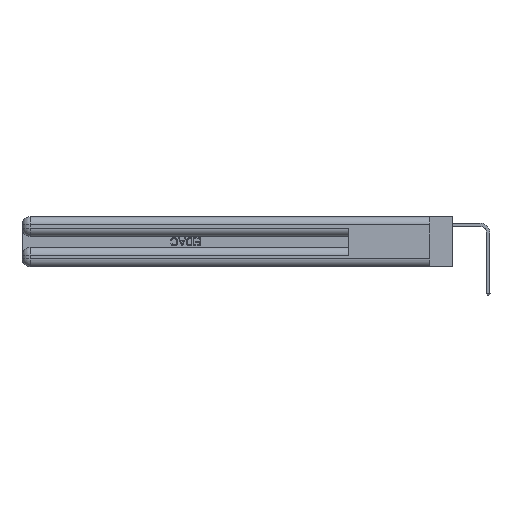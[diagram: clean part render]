
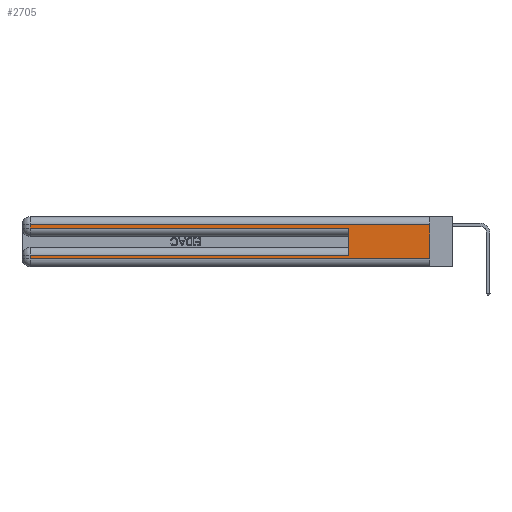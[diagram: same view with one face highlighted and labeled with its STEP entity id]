
A CAD part, left-side view. The second image highlights one B-rep face of the part: STEP entity #2705.
In plain terms, the highlighted planar face has unit normal (-1, 0, 0).
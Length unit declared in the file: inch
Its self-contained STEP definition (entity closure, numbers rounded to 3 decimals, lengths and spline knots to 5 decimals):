
#549 = LINE ( 'NONE', #13289, #26780 ) ;
#654 = CARTESIAN_POINT ( 'NONE',  ( 0., 0., 0.31 ) ) ;
#1462 = EDGE_CURVE ( 'NONE', #16318, #24122, #12923, .T. ) ;
#1870 = EDGE_LOOP ( 'NONE', ( #3384, #30017, #4647, #6444, #7582, #5738, #4512, #25020 ) ) ;
#2015 = EDGE_CURVE ( 'NONE', #24122, #26317, #24005, .T. ) ;
#2305 = VERTEX_POINT ( 'NONE', #14566 ) ;
#2485 = EDGE_CURVE ( 'NONE', #26317, #19376, #29432, .T. ) ;
#2705 = ADVANCED_FACE ( 'NONE', ( #11775 ), #16457, .F. ) ;
#2742 = VECTOR ( 'NONE', #7947, 39.37008 ) ;
#2922 = DIRECTION ( 'NONE',  ( 0., -1., 0. ) ) ;
#3250 = CARTESIAN_POINT ( 'NONE',  ( 0., 2.94, 0.37 ) ) ;
#3368 = CARTESIAN_POINT ( 'NONE',  ( 0., 0.6, 0.285 ) ) ;
#3384 = ORIENTED_EDGE ( 'NONE', *, *, #27199, .F. ) ;
#3673 = CARTESIAN_POINT ( 'NONE',  ( 0., 2.94, 0.37 ) ) ;
#3937 = EDGE_CURVE ( 'NONE', #23495, #30847, #549, .T. ) ;
#4512 = ORIENTED_EDGE ( 'NONE', *, *, #18776, .T. ) ;
#4647 = ORIENTED_EDGE ( 'NONE', *, *, #2015, .T. ) ;
#5738 = ORIENTED_EDGE ( 'NONE', *, *, #3937, .T. ) ;
#6089 = DIRECTION ( 'NONE',  ( 0., -1., 0. ) ) ;
#6444 = ORIENTED_EDGE ( 'NONE', *, *, #2485, .T. ) ;
#6616 = CARTESIAN_POINT ( 'NONE',  ( 0., 0.6, 0.085 ) ) ;
#7582 = ORIENTED_EDGE ( 'NONE', *, *, #7604, .F. ) ;
#7604 = EDGE_CURVE ( 'NONE', #23495, #19376, #28456, .T. ) ;
#7947 = DIRECTION ( 'NONE',  ( 0., 0., -1. ) ) ;
#8620 = VECTOR ( 'NONE', #2922, 39.37008 ) ;
#9493 = DIRECTION ( 'NONE',  ( 1., 0., 0. ) ) ;
#10477 = DIRECTION ( 'NONE',  ( 0., 1., 0. ) ) ;
#11453 = DIRECTION ( 'NONE',  ( 0., 0., -1. ) ) ;
#11775 = FACE_OUTER_BOUND ( 'NONE', #1870, .T. ) ;
#12232 = VECTOR ( 'NONE', #22941, 39.37008 ) ;
#12923 = LINE ( 'NONE', #654, #22293 ) ;
#12926 = VECTOR ( 'NONE', #18756, 39.37008 ) ;
#13289 = CARTESIAN_POINT ( 'NONE',  ( 0., 0., 0.085 ) ) ;
#14566 = CARTESIAN_POINT ( 'NONE',  ( 0., 2.94, 0.06 ) ) ;
#14877 = CARTESIAN_POINT ( 'NONE',  ( 0., 0., 0.285 ) ) ;
#16159 = CARTESIAN_POINT ( 'NONE',  ( 0., 0.6, 0.145 ) ) ;
#16318 = VERTEX_POINT ( 'NONE', #19043 ) ;
#16457 = PLANE ( 'NONE',  #22047 ) ;
#18538 = CARTESIAN_POINT ( 'NONE',  ( 0., 0., 0.06 ) ) ;
#18756 = DIRECTION ( 'NONE',  ( 0., 0., 1. ) ) ;
#18776 = EDGE_CURVE ( 'NONE', #30847, #2305, #25368, .T. ) ;
#19043 = CARTESIAN_POINT ( 'NONE',  ( 0., 0., 0.31 ) ) ;
#19266 = VERTEX_POINT ( 'NONE', #31570 ) ;
#19376 = VERTEX_POINT ( 'NONE', #3368 ) ;
#19891 = CARTESIAN_POINT ( 'NONE',  ( 0., 2.94, 0.285 ) ) ;
#21432 = LINE ( 'NONE', #18538, #23248 ) ;
#22047 = AXIS2_PLACEMENT_3D ( 'NONE', #23899, #9493, #11453 ) ;
#22293 = VECTOR ( 'NONE', #10477, 39.37008 ) ;
#22941 = DIRECTION ( 'NONE',  ( 0., 0., -1. ) ) ;
#23138 = DIRECTION ( 'NONE',  ( 0., 1., 0. ) ) ;
#23248 = VECTOR ( 'NONE', #6089, 39.37008 ) ;
#23495 = VERTEX_POINT ( 'NONE', #6616 ) ;
#23899 = CARTESIAN_POINT ( 'NONE',  ( 0., 0., 0.37 ) ) ;
#24005 = LINE ( 'NONE', #3673, #24090 ) ;
#24090 = VECTOR ( 'NONE', #28388, 39.37008 ) ;
#24122 = VERTEX_POINT ( 'NONE', #24651 ) ;
#24651 = CARTESIAN_POINT ( 'NONE',  ( 0., 2.94, 0.31 ) ) ;
#25020 = ORIENTED_EDGE ( 'NONE', *, *, #25114, .T. ) ;
#25114 = EDGE_CURVE ( 'NONE', #2305, #19266, #21432, .T. ) ;
#25368 = LINE ( 'NONE', #3250, #12232 ) ;
#26317 = VERTEX_POINT ( 'NONE', #19891 ) ;
#26780 = VECTOR ( 'NONE', #23138, 39.37008 ) ;
#27199 = EDGE_CURVE ( 'NONE', #16318, #19266, #30256, .T. ) ;
#28092 = CARTESIAN_POINT ( 'NONE',  ( 0., 2.94, 0.085 ) ) ;
#28388 = DIRECTION ( 'NONE',  ( 0., 0., -1. ) ) ;
#28456 = LINE ( 'NONE', #16159, #12926 ) ;
#29432 = LINE ( 'NONE', #14877, #8620 ) ;
#29952 = CARTESIAN_POINT ( 'NONE',  ( 0., 0., 0.37 ) ) ;
#30017 = ORIENTED_EDGE ( 'NONE', *, *, #1462, .T. ) ;
#30256 = LINE ( 'NONE', #29952, #2742 ) ;
#30847 = VERTEX_POINT ( 'NONE', #28092 ) ;
#31570 = CARTESIAN_POINT ( 'NONE',  ( 0., 0., 0.06 ) ) ;
